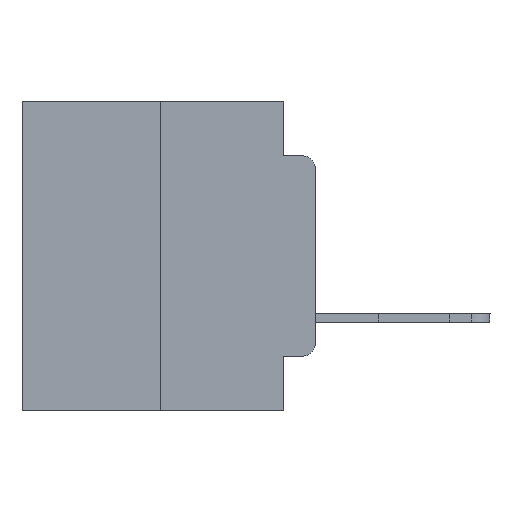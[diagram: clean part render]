
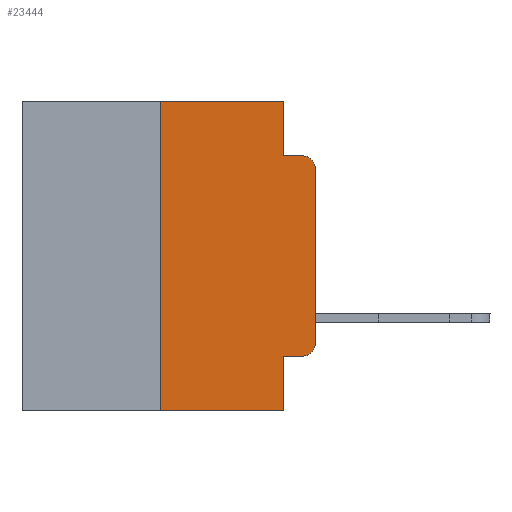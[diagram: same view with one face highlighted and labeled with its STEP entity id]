
A CAD part, left-side view. The second image highlights one B-rep face of the part: STEP entity #23444.
In plain terms, the highlighted planar face has unit normal (-1, 0, 0).
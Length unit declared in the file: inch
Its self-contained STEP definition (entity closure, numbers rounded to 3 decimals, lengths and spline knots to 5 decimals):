
#1158 = ORIENTED_EDGE ( 'NONE', *, *, #9259, .F. ) ;
#1203 = CARTESIAN_POINT ( 'NONE',  ( 0., 0.25, 0. ) ) ;
#1279 = CARTESIAN_POINT ( 'NONE',  ( 0., 0., 0. ) ) ;
#1442 = VERTEX_POINT ( 'NONE', #18308 ) ;
#1712 = CARTESIAN_POINT ( 'NONE',  ( 0., 0.051, 0. ) ) ;
#1990 = ORIENTED_EDGE ( 'NONE', *, *, #2603, .T. ) ;
#2481 = VECTOR ( 'NONE', #21665, 39.37008 ) ;
#2603 = EDGE_CURVE ( 'NONE', #1442, #3816, #15117, .T. ) ;
#2678 = DIRECTION ( 'NONE',  ( 0., 0., -1. ) ) ;
#2695 = VECTOR ( 'NONE', #2751, 39.37008 ) ;
#2751 = DIRECTION ( 'NONE',  ( 0., 0., -1. ) ) ;
#2930 = ORIENTED_EDGE ( 'NONE', *, *, #22331, .T. ) ;
#3461 = DIRECTION ( 'NONE',  ( 0., 0., 1. ) ) ;
#3816 = VERTEX_POINT ( 'NONE', #7312 ) ;
#4595 = VERTEX_POINT ( 'NONE', #12207 ) ;
#4642 = ORIENTED_EDGE ( 'NONE', *, *, #26725, .F. ) ;
#4660 = DIRECTION ( 'NONE',  ( 0., -1., 0. ) ) ;
#4686 = DIRECTION ( 'NONE',  ( 0., 0., -1. ) ) ;
#4757 = LINE ( 'NONE', #26883, #9632 ) ;
#4800 = CIRCLE ( 'NONE', #12550, 0.02 ) ;
#5273 = ORIENTED_EDGE ( 'NONE', *, *, #6044, .T. ) ;
#5855 = DIRECTION ( 'NONE',  ( 0., -1., 0. ) ) ;
#6044 = EDGE_CURVE ( 'NONE', #3816, #24358, #4800, .T. ) ;
#6484 = PLANE ( 'NONE',  #25528 ) ;
#6589 = LINE ( 'NONE', #6895, #2695 ) ;
#6594 = VECTOR ( 'NONE', #19885, 39.37008 ) ;
#6895 = CARTESIAN_POINT ( 'NONE',  ( 0., 0.051, 0. ) ) ;
#7312 = CARTESIAN_POINT ( 'NONE',  ( 0., 0.02, -0.4115 ) ) ;
#7630 = CARTESIAN_POINT ( 'NONE',  ( 0., 0.02, -0.1085 ) ) ;
#7826 = DIRECTION ( 'NONE',  ( 0., -1., 0. ) ) ;
#7845 = LINE ( 'NONE', #23530, #15967 ) ;
#7865 = VECTOR ( 'NONE', #3461, 39.37008 ) ;
#9051 = ORIENTED_EDGE ( 'NONE', *, *, #16796, .T. ) ;
#9259 = EDGE_CURVE ( 'NONE', #12092, #4595, #15913, .T. ) ;
#9632 = VECTOR ( 'NONE', #7826, 39.37008 ) ;
#9865 = VERTEX_POINT ( 'NONE', #11611 ) ;
#10360 = VECTOR ( 'NONE', #4686, 39.37008 ) ;
#11497 = CARTESIAN_POINT ( 'NONE',  ( 0., 0., -0.1085 ) ) ;
#11529 = VECTOR ( 'NONE', #5855, 39.37008 ) ;
#11611 = CARTESIAN_POINT ( 'NONE',  ( 0., 0.051, -0.5 ) ) ;
#11773 = EDGE_CURVE ( 'NONE', #14676, #12092, #20663, .T. ) ;
#12092 = VERTEX_POINT ( 'NONE', #1712 ) ;
#12207 = CARTESIAN_POINT ( 'NONE',  ( 0., 0.051, -0.0885 ) ) ;
#12463 = ORIENTED_EDGE ( 'NONE', *, *, #11773, .F. ) ;
#12550 = AXIS2_PLACEMENT_3D ( 'NONE', #19215, #15123, #2678 ) ;
#12586 = EDGE_CURVE ( 'NONE', #24768, #25093, #16084, .T. ) ;
#12932 = EDGE_LOOP ( 'NONE', ( #9051, #14020, #15883, #1158, #12463, #4642, #2930, #21370, #1990, #5273 ) ) ;
#13026 = CARTESIAN_POINT ( 'NONE',  ( 0., 0.473, 0. ) ) ;
#13098 = DIRECTION ( 'NONE',  ( 1., 0., 0. ) ) ;
#14020 = ORIENTED_EDGE ( 'NONE', *, *, #12586, .T. ) ;
#14676 = VERTEX_POINT ( 'NONE', #1203 ) ;
#15117 = LINE ( 'NONE', #22399, #11529 ) ;
#15123 = DIRECTION ( 'NONE',  ( -1., 0., 0. ) ) ;
#15303 = DIRECTION ( 'NONE',  ( 0., 0., -1. ) ) ;
#15704 = LINE ( 'NONE', #17830, #6594 ) ;
#15883 = ORIENTED_EDGE ( 'NONE', *, *, #25309, .F. ) ;
#15913 = LINE ( 'NONE', #19240, #10360 ) ;
#15967 = VECTOR ( 'NONE', #4660, 39.37008 ) ;
#16084 = CIRCLE ( 'NONE', #18439, 0.02 ) ;
#16796 = EDGE_CURVE ( 'NONE', #24358, #24768, #16993, .T. ) ;
#16993 = LINE ( 'NONE', #1279, #7865 ) ;
#17318 = CARTESIAN_POINT ( 'NONE',  ( 0., 0.473, 0. ) ) ;
#17674 = DIRECTION ( 'NONE',  ( -1., 0., 0. ) ) ;
#17830 = CARTESIAN_POINT ( 'NONE',  ( 0., 0.25, 0. ) ) ;
#18308 = CARTESIAN_POINT ( 'NONE',  ( 0., 0.051, -0.4115 ) ) ;
#18439 = AXIS2_PLACEMENT_3D ( 'NONE', #7630, #17674, #26433 ) ;
#18791 = CARTESIAN_POINT ( 'NONE',  ( 0., 0.25, -0.5 ) ) ;
#19215 = CARTESIAN_POINT ( 'NONE',  ( 0., 0.02, -0.3915 ) ) ;
#19240 = CARTESIAN_POINT ( 'NONE',  ( 0., 0.051, 0. ) ) ;
#19885 = DIRECTION ( 'NONE',  ( 0., 0., 1. ) ) ;
#20663 = LINE ( 'NONE', #13026, #2481 ) ;
#20930 = CARTESIAN_POINT ( 'NONE',  ( 0., 0.02, -0.0885 ) ) ;
#21370 = ORIENTED_EDGE ( 'NONE', *, *, #26039, .F. ) ;
#21665 = DIRECTION ( 'NONE',  ( 0., -1., 0. ) ) ;
#21920 = FACE_OUTER_BOUND ( 'NONE', #12932, .T. ) ;
#22331 = EDGE_CURVE ( 'NONE', #25149, #9865, #4757, .T. ) ;
#22399 = CARTESIAN_POINT ( 'NONE',  ( 0., 0.051, -0.4115 ) ) ;
#22691 = CARTESIAN_POINT ( 'NONE',  ( 0., 0., -0.3915 ) ) ;
#23444 = ADVANCED_FACE ( 'NONE', ( #21920 ), #6484, .F. ) ;
#23530 = CARTESIAN_POINT ( 'NONE',  ( 0., 0.051, -0.0885 ) ) ;
#24358 = VERTEX_POINT ( 'NONE', #22691 ) ;
#24768 = VERTEX_POINT ( 'NONE', #11497 ) ;
#25093 = VERTEX_POINT ( 'NONE', #20930 ) ;
#25149 = VERTEX_POINT ( 'NONE', #18791 ) ;
#25309 = EDGE_CURVE ( 'NONE', #4595, #25093, #7845, .T. ) ;
#25528 = AXIS2_PLACEMENT_3D ( 'NONE', #17318, #13098, #15303 ) ;
#26039 = EDGE_CURVE ( 'NONE', #1442, #9865, #6589, .T. ) ;
#26433 = DIRECTION ( 'NONE',  ( 0., 0., -1. ) ) ;
#26725 = EDGE_CURVE ( 'NONE', #25149, #14676, #15704, .T. ) ;
#26883 = CARTESIAN_POINT ( 'NONE',  ( 0., 0.473, -0.5 ) ) ;
